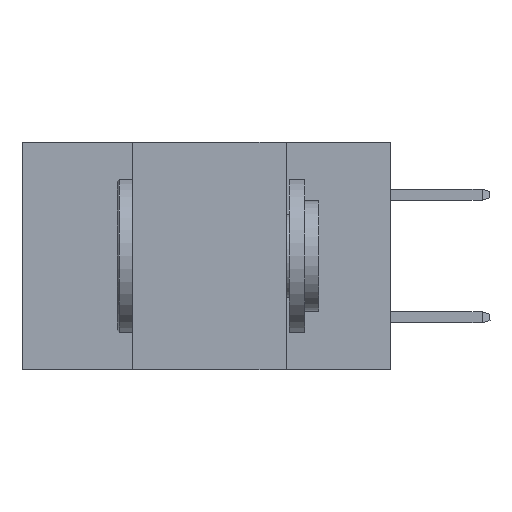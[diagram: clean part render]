
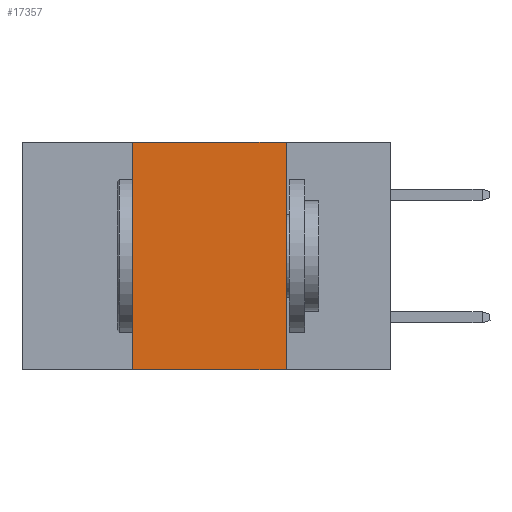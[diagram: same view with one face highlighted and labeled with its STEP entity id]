
A CAD part, left-side view. The second image highlights one B-rep face of the part: STEP entity #17357.
In plain terms, the highlighted planar face has unit normal (-1, 0, 0).
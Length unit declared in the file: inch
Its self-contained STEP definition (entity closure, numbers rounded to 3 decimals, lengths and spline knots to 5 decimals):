
#97 = LINE ( 'NONE', #8127, #15349 ) ;
#668 = EDGE_CURVE ( 'NONE', #1989, #13852, #97, .T. ) ;
#1039 = CARTESIAN_POINT ( 'NONE',  ( 0., 0.6, 0. ) ) ;
#1057 = LINE ( 'NONE', #14543, #5060 ) ;
#1372 = AXIS2_PLACEMENT_3D ( 'NONE', #1039, #2615, #12593 ) ;
#1989 = VERTEX_POINT ( 'NONE', #14905 ) ;
#2020 = EDGE_CURVE ( 'NONE', #17254, #13889, #1057, .T. ) ;
#2615 = DIRECTION ( 'NONE',  ( 1., 0., 0. ) ) ;
#4335 = LINE ( 'NONE', #16169, #12325 ) ;
#5060 = VECTOR ( 'NONE', #14638, 39.37008 ) ;
#5246 = CARTESIAN_POINT ( 'NONE',  ( 0., 0.42, -0.37 ) ) ;
#6976 = LINE ( 'NONE', #17704, #10350 ) ;
#7784 = DIRECTION ( 'NONE',  ( 0., -1., 0. ) ) ;
#8036 = DIRECTION ( 'NONE',  ( 0., 0., -1. ) ) ;
#8127 = CARTESIAN_POINT ( 'NONE',  ( 0., 0.6, 0. ) ) ;
#8279 = ORIENTED_EDGE ( 'NONE', *, *, #18070, .F. ) ;
#10350 = VECTOR ( 'NONE', #11153, 39.37008 ) ;
#11061 = CARTESIAN_POINT ( 'NONE',  ( 0., 0.17, -0.37 ) ) ;
#11153 = DIRECTION ( 'NONE',  ( 0., 0., 1. ) ) ;
#11329 = ORIENTED_EDGE ( 'NONE', *, *, #15926, .F. ) ;
#12325 = VECTOR ( 'NONE', #8036, 39.37008 ) ;
#12593 = DIRECTION ( 'NONE',  ( 0., 0., -1. ) ) ;
#13852 = VERTEX_POINT ( 'NONE', #17497 ) ;
#13889 = VERTEX_POINT ( 'NONE', #11061 ) ;
#14543 = CARTESIAN_POINT ( 'NONE',  ( 0., 0.6, -0.37 ) ) ;
#14638 = DIRECTION ( 'NONE',  ( 0., -1., 0. ) ) ;
#14769 = EDGE_LOOP ( 'NONE', ( #11329, #14894, #8279, #15521 ) ) ;
#14894 = ORIENTED_EDGE ( 'NONE', *, *, #668, .F. ) ;
#14905 = CARTESIAN_POINT ( 'NONE',  ( 0., 0.42, 0. ) ) ;
#15349 = VECTOR ( 'NONE', #7784, 39.37008 ) ;
#15521 = ORIENTED_EDGE ( 'NONE', *, *, #2020, .T. ) ;
#15566 = FACE_OUTER_BOUND ( 'NONE', #14769, .T. ) ;
#15926 = EDGE_CURVE ( 'NONE', #13852, #13889, #4335, .T. ) ;
#16169 = CARTESIAN_POINT ( 'NONE',  ( 0., 0.17, 0. ) ) ;
#17254 = VERTEX_POINT ( 'NONE', #5246 ) ;
#17357 = ADVANCED_FACE ( 'NONE', ( #15566 ), #17800, .F. ) ;
#17497 = CARTESIAN_POINT ( 'NONE',  ( 0., 0.17, 0. ) ) ;
#17704 = CARTESIAN_POINT ( 'NONE',  ( 0., 0.42, 0. ) ) ;
#17800 = PLANE ( 'NONE',  #1372 ) ;
#18070 = EDGE_CURVE ( 'NONE', #17254, #1989, #6976, .T. ) ;
